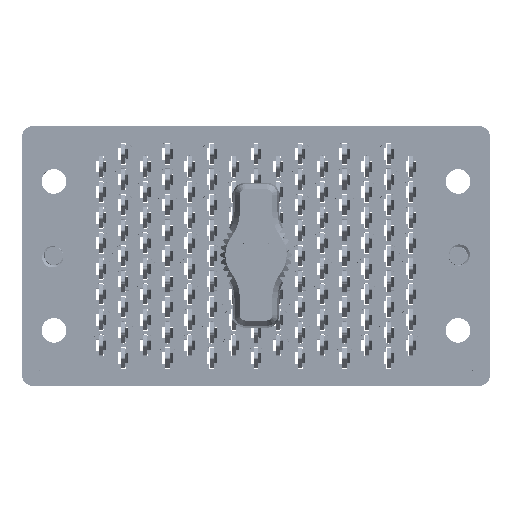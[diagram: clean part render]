
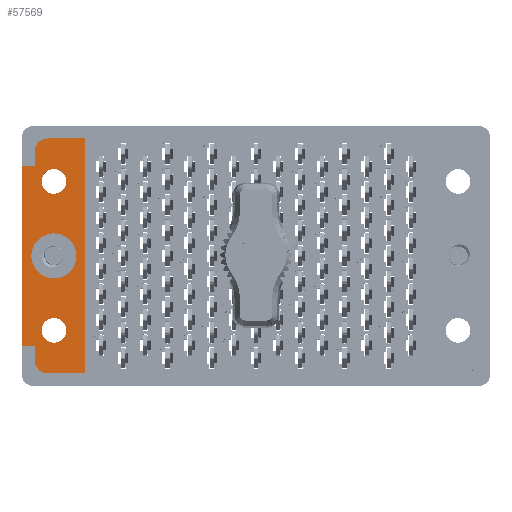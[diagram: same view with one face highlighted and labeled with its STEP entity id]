
A CAD part, top view. The second image highlights one B-rep face of the part: STEP entity #57569.
In plain terms, the highlighted planar face has unit normal (0, 0, 1).
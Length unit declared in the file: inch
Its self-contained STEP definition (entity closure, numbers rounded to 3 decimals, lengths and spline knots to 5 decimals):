
#174 = ORIENTED_EDGE ( 'NONE', *, *, #75521, .T. ) ;
#2536 = VECTOR ( 'NONE', #72771, 39.37008 ) ;
#2749 = CARTESIAN_POINT ( 'NONE',  ( -1.1875, 0.4375, -0.117 ) ) ;
#3541 = CARTESIAN_POINT ( 'NONE',  ( 0., -0.5285, -0.117 ) ) ;
#5200 = EDGE_CURVE ( 'NONE', #87564, #110331, #85868, .T. ) ;
#5232 = EDGE_CURVE ( 'NONE', #27044, #77374, #83053, .T. ) ;
#5413 = CARTESIAN_POINT ( 'NONE',  ( -1.005, 0.69, -0.117 ) ) ;
#5790 = CARTESIAN_POINT ( 'NONE',  ( -1.375, -0.5285, -0.117 ) ) ;
#6864 = EDGE_CURVE ( 'NONE', #79090, #12664, #71406, .T. ) ;
#7177 = FACE_BOUND ( 'NONE', #95284, .T. ) ;
#7418 = VERTEX_POINT ( 'NONE', #64014 ) ;
#10234 = CIRCLE ( 'NONE', #84095, 0.0725 ) ;
#11903 = CARTESIAN_POINT ( 'NONE',  ( -1.1875, 0., -0.117 ) ) ;
#12664 = VERTEX_POINT ( 'NONE', #116550 ) ;
#13829 = VECTOR ( 'NONE', #111520, 39.37008 ) ;
#14508 = ORIENTED_EDGE ( 'NONE', *, *, #5232, .F. ) ;
#15708 = AXIS2_PLACEMENT_3D ( 'NONE', #46441, #83471, #92096 ) ;
#17310 = CARTESIAN_POINT ( 'NONE',  ( -1.3, 0., -0.117 ) ) ;
#17365 = VERTEX_POINT ( 'NONE', #24144 ) ;
#21188 = DIRECTION ( 'NONE',  ( -1., 0., 0. ) ) ;
#21520 = ORIENTED_EDGE ( 'NONE', *, *, #92613, .T. ) ;
#21679 = EDGE_CURVE ( 'NONE', #27390, #109313, #46058, .T. ) ;
#22453 = DIRECTION ( 'NONE',  ( 0., 0., 1. ) ) ;
#23219 = DIRECTION ( 'NONE',  ( 1., 0., 0. ) ) ;
#24144 = CARTESIAN_POINT ( 'NONE',  ( -1.3, -0.615, -0.117 ) ) ;
#24171 = CARTESIAN_POINT ( 'NONE',  ( -1.375, 0.7625, -0.117 ) ) ;
#25982 = ORIENTED_EDGE ( 'NONE', *, *, #5200, .F. ) ;
#26823 = EDGE_CURVE ( 'NONE', #12664, #88238, #113839, .T. ) ;
#27044 = VERTEX_POINT ( 'NONE', #103196 ) ;
#27390 = VERTEX_POINT ( 'NONE', #89400 ) ;
#29157 = CARTESIAN_POINT ( 'NONE',  ( -1.26, -0.4375, -0.117 ) ) ;
#30980 = ORIENTED_EDGE ( 'NONE', *, *, #96116, .F. ) ;
#31079 = DIRECTION ( 'NONE',  ( 0., 0., 1. ) ) ;
#31862 = VERTEX_POINT ( 'NONE', #43621 ) ;
#32437 = AXIS2_PLACEMENT_3D ( 'NONE', #53079, #105842, #80309 ) ;
#32566 = AXIS2_PLACEMENT_3D ( 'NONE', #108921, #73911, #65623 ) ;
#32661 = EDGE_CURVE ( 'NONE', #27044, #17365, #86639, .T. ) ;
#33030 = AXIS2_PLACEMENT_3D ( 'NONE', #57870, #31079, #94036 ) ;
#33620 = LINE ( 'NONE', #24171, #36411 ) ;
#33800 = ORIENTED_EDGE ( 'NONE', *, *, #6864, .T. ) ;
#34886 = CARTESIAN_POINT ( 'NONE',  ( -1.3, 0.5285, -0.117 ) ) ;
#36411 = VECTOR ( 'NONE', #51295, 39.37008 ) ;
#39754 = DIRECTION ( 'NONE',  ( -1., 0., 0. ) ) ;
#41278 = CARTESIAN_POINT ( 'NONE',  ( -1.055, 0., -0.117 ) ) ;
#41331 = CARTESIAN_POINT ( 'NONE',  ( -1.1875, -0.4375, -0.117 ) ) ;
#42630 = LINE ( 'NONE', #78633, #72233 ) ;
#43621 = CARTESIAN_POINT ( 'NONE',  ( -1.32, 0., -0.117 ) ) ;
#43949 = AXIS2_PLACEMENT_3D ( 'NONE', #104367, #86321, #111905 ) ;
#44120 = ORIENTED_EDGE ( 'NONE', *, *, #88082, .T. ) ;
#44609 = ORIENTED_EDGE ( 'NONE', *, *, #45733, .F. ) ;
#45733 = EDGE_CURVE ( 'NONE', #31862, #79078, #83124, .T. ) ;
#46035 = EDGE_CURVE ( 'NONE', #113326, #7418, #101332, .T. ) ;
#46058 = CIRCLE ( 'NONE', #113346, 0.0725 ) ;
#46369 = CIRCLE ( 'NONE', #60612, 0.1325 ) ;
#46441 = CARTESIAN_POINT ( 'NONE',  ( -1.1875, 0., -0.117 ) ) ;
#47817 = VECTOR ( 'NONE', #95560, 39.37008 ) ;
#48341 = EDGE_LOOP ( 'NONE', ( #108196, #44609 ) ) ;
#48548 = VECTOR ( 'NONE', #62329, 39.37008 ) ;
#49088 = CARTESIAN_POINT ( 'NONE',  ( 0., 0.69, -0.117 ) ) ;
#49301 = CARTESIAN_POINT ( 'NONE',  ( 0., 0.5285, -0.117 ) ) ;
#50166 = CIRCLE ( 'NONE', #32566, 0.075 ) ;
#50292 = CARTESIAN_POINT ( 'NONE',  ( 0., -0.69, -0.117 ) ) ;
#50398 = EDGE_CURVE ( 'NONE', #109313, #27390, #91371, .T. ) ;
#51295 = DIRECTION ( 'NONE',  ( 0., -1., 0. ) ) ;
#51664 = ORIENTED_EDGE ( 'NONE', *, *, #21679, .F. ) ;
#53079 = CARTESIAN_POINT ( 'NONE',  ( -1.375, -0.7625, -0.117 ) ) ;
#53526 = VERTEX_POINT ( 'NONE', #72922 ) ;
#54600 = LINE ( 'NONE', #49301, #13829 ) ;
#55058 = FACE_BOUND ( 'NONE', #88869, .T. ) ;
#55503 = DIRECTION ( 'NONE',  ( 0., 0., 1. ) ) ;
#55916 = VECTOR ( 'NONE', #21188, 39.37008 ) ;
#57569 = ADVANCED_FACE ( 'NONE', ( #55058, #7177, #100101, #70557 ), #78743, .T. ) ;
#57870 = CARTESIAN_POINT ( 'NONE',  ( -1.1875, -0.4375, -0.117 ) ) ;
#60612 = AXIS2_PLACEMENT_3D ( 'NONE', #11903, #76450, #92598 ) ;
#62074 = ORIENTED_EDGE ( 'NONE', *, *, #103558, .T. ) ;
#62329 = DIRECTION ( 'NONE',  ( 0., -1., 0. ) ) ;
#64014 = CARTESIAN_POINT ( 'NONE',  ( -1.225, -0.69, -0.117 ) ) ;
#65623 = DIRECTION ( 'NONE',  ( 1., 0., 0. ) ) ;
#66338 = VERTEX_POINT ( 'NONE', #34886 ) ;
#70217 = CARTESIAN_POINT ( 'NONE',  ( -1.005, -0.69, -0.117 ) ) ;
#70557 = FACE_OUTER_BOUND ( 'NONE', #83520, .T. ) ;
#71229 = CARTESIAN_POINT ( 'NONE',  ( -1.3, 0.615, -0.117 ) ) ;
#71406 = LINE ( 'NONE', #49088, #55916 ) ;
#71449 = AXIS2_PLACEMENT_3D ( 'NONE', #74150, #91850, #109535 ) ;
#72233 = VECTOR ( 'NONE', #114839, 39.37008 ) ;
#72771 = DIRECTION ( 'NONE',  ( 0., -1., 0. ) ) ;
#72922 = CARTESIAN_POINT ( 'NONE',  ( -1.375, 0.5285, -0.117 ) ) ;
#73911 = DIRECTION ( 'NONE',  ( 0., 0., 1. ) ) ;
#74027 = ORIENTED_EDGE ( 'NONE', *, *, #46035, .F. ) ;
#74150 = CARTESIAN_POINT ( 'NONE',  ( -1.225, 0.615, -0.117 ) ) ;
#75521 = EDGE_CURVE ( 'NONE', #17365, #7418, #50166, .T. ) ;
#76450 = DIRECTION ( 'NONE',  ( 0., 0., 1. ) ) ;
#77374 = VERTEX_POINT ( 'NONE', #5790 ) ;
#78633 = CARTESIAN_POINT ( 'NONE',  ( -1.005, 0.7625, -0.117 ) ) ;
#78743 = PLANE ( 'NONE',  #32437 ) ;
#79078 = VERTEX_POINT ( 'NONE', #41278 ) ;
#79090 = VERTEX_POINT ( 'NONE', #5413 ) ;
#80309 = DIRECTION ( 'NONE',  ( 1., 0., 0. ) ) ;
#81820 = EDGE_CURVE ( 'NONE', #79078, #31862, #46369, .T. ) ;
#83053 = LINE ( 'NONE', #3541, #105950 ) ;
#83124 = CIRCLE ( 'NONE', #15708, 0.1325 ) ;
#83471 = DIRECTION ( 'NONE',  ( 0., 0., 1. ) ) ;
#83520 = EDGE_LOOP ( 'NONE', ( #33800, #101631, #97595, #62074, #44120, #14508, #92355, #174, #74027, #21520 ) ) ;
#84095 = AXIS2_PLACEMENT_3D ( 'NONE', #41331, #22453, #23219 ) ;
#85868 = CIRCLE ( 'NONE', #33030, 0.0725 ) ;
#86321 = DIRECTION ( 'NONE',  ( 0., 0., 1. ) ) ;
#86639 = LINE ( 'NONE', #110343, #48548 ) ;
#87564 = VERTEX_POINT ( 'NONE', #111814 ) ;
#88082 = EDGE_CURVE ( 'NONE', #53526, #77374, #33620, .T. ) ;
#88238 = VERTEX_POINT ( 'NONE', #71229 ) ;
#88869 = EDGE_LOOP ( 'NONE', ( #109680, #51664 ) ) ;
#89400 = CARTESIAN_POINT ( 'NONE',  ( -1.115, 0.4375, -0.117 ) ) ;
#91371 = CIRCLE ( 'NONE', #43949, 0.0725 ) ;
#91850 = DIRECTION ( 'NONE',  ( 0., 0., 1. ) ) ;
#92096 = DIRECTION ( 'NONE',  ( 1., 0., 0. ) ) ;
#92101 = DIRECTION ( 'NONE',  ( 1., 0., 0. ) ) ;
#92355 = ORIENTED_EDGE ( 'NONE', *, *, #32661, .T. ) ;
#92598 = DIRECTION ( 'NONE',  ( 1., 0., 0. ) ) ;
#92613 = EDGE_CURVE ( 'NONE', #113326, #79090, #42630, .T. ) ;
#94036 = DIRECTION ( 'NONE',  ( 1., 0., 0. ) ) ;
#95284 = EDGE_LOOP ( 'NONE', ( #30980, #25982 ) ) ;
#95560 = DIRECTION ( 'NONE',  ( -1., 0., 0. ) ) ;
#96116 = EDGE_CURVE ( 'NONE', #110331, #87564, #10234, .T. ) ;
#97595 = ORIENTED_EDGE ( 'NONE', *, *, #116049, .T. ) ;
#100101 = FACE_BOUND ( 'NONE', #48341, .T. ) ;
#101093 = LINE ( 'NONE', #17310, #2536 ) ;
#101332 = LINE ( 'NONE', #50292, #47817 ) ;
#101631 = ORIENTED_EDGE ( 'NONE', *, *, #26823, .T. ) ;
#103196 = CARTESIAN_POINT ( 'NONE',  ( -1.3, -0.5285, -0.117 ) ) ;
#103558 = EDGE_CURVE ( 'NONE', #66338, #53526, #54600, .T. ) ;
#104367 = CARTESIAN_POINT ( 'NONE',  ( -1.1875, 0.4375, -0.117 ) ) ;
#105842 = DIRECTION ( 'NONE',  ( 0., 0., 1. ) ) ;
#105950 = VECTOR ( 'NONE', #39754, 39.37008 ) ;
#108196 = ORIENTED_EDGE ( 'NONE', *, *, #81820, .F. ) ;
#108921 = CARTESIAN_POINT ( 'NONE',  ( -1.225, -0.615, -0.117 ) ) ;
#109313 = VERTEX_POINT ( 'NONE', #111278 ) ;
#109535 = DIRECTION ( 'NONE',  ( 1., 0., 0. ) ) ;
#109680 = ORIENTED_EDGE ( 'NONE', *, *, #50398, .F. ) ;
#110331 = VERTEX_POINT ( 'NONE', #29157 ) ;
#110343 = CARTESIAN_POINT ( 'NONE',  ( -1.3, 0., -0.117 ) ) ;
#111278 = CARTESIAN_POINT ( 'NONE',  ( -1.26, 0.4375, -0.117 ) ) ;
#111520 = DIRECTION ( 'NONE',  ( -1., 0., 0. ) ) ;
#111814 = CARTESIAN_POINT ( 'NONE',  ( -1.115, -0.4375, -0.117 ) ) ;
#111905 = DIRECTION ( 'NONE',  ( 1., 0., 0. ) ) ;
#113326 = VERTEX_POINT ( 'NONE', #70217 ) ;
#113346 = AXIS2_PLACEMENT_3D ( 'NONE', #2749, #55503, #92101 ) ;
#113839 = CIRCLE ( 'NONE', #71449, 0.075 ) ;
#114839 = DIRECTION ( 'NONE',  ( 0., 1., 0. ) ) ;
#116049 = EDGE_CURVE ( 'NONE', #88238, #66338, #101093, .T. ) ;
#116550 = CARTESIAN_POINT ( 'NONE',  ( -1.225, 0.69, -0.117 ) ) ;
